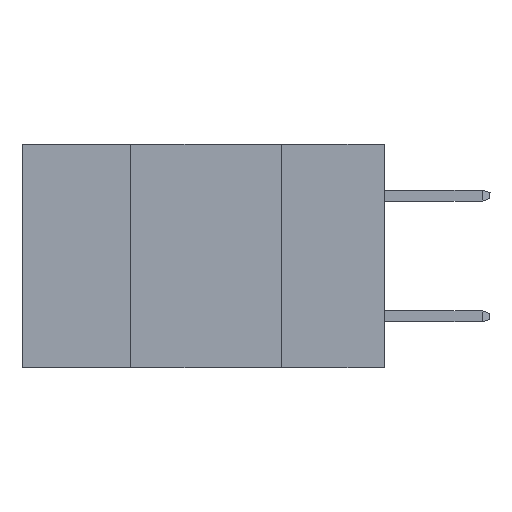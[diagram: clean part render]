
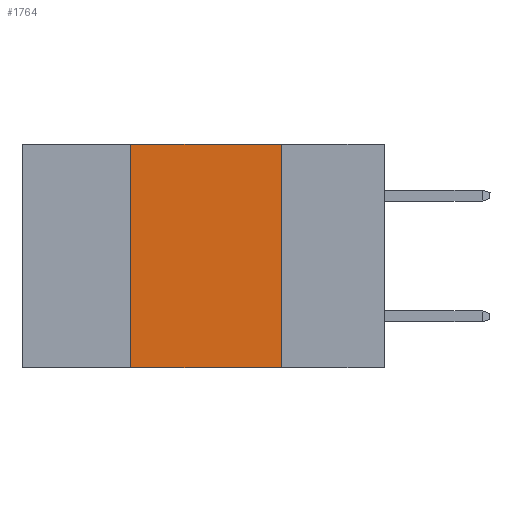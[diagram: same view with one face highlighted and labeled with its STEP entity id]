
A CAD part, left-side view. The second image highlights one B-rep face of the part: STEP entity #1764.
In plain terms, the highlighted planar face has unit normal (-1, 0, 0).
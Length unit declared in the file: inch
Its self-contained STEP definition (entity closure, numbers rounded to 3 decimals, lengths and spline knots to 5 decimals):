
#1295 = VERTEX_POINT ( 'NONE', #20306 ) ;
#1764 = ADVANCED_FACE ( 'NONE', ( #6609 ), #15879, .F. ) ;
#3028 = CARTESIAN_POINT ( 'NONE',  ( 0., 0.17, -0.37 ) ) ;
#3430 = ORIENTED_EDGE ( 'NONE', *, *, #4189, .F. ) ;
#3441 = CARTESIAN_POINT ( 'NONE',  ( 0., 0.42, -0.37 ) ) ;
#4189 = EDGE_CURVE ( 'NONE', #1295, #16465, #11173, .T. ) ;
#4490 = DIRECTION ( 'NONE',  ( 0., 0., -1. ) ) ;
#4942 = DIRECTION ( 'NONE',  ( 0., 0., 1. ) ) ;
#6105 = CARTESIAN_POINT ( 'NONE',  ( 0., 0.6, 0. ) ) ;
#6609 = FACE_OUTER_BOUND ( 'NONE', #9655, .T. ) ;
#7388 = VERTEX_POINT ( 'NONE', #3441 ) ;
#8263 = EDGE_CURVE ( 'NONE', #16465, #20107, #13062, .T. ) ;
#9372 = DIRECTION ( 'NONE',  ( 0., -1., 0. ) ) ;
#9398 = DIRECTION ( 'NONE',  ( 1., 0., 0. ) ) ;
#9655 = EDGE_LOOP ( 'NONE', ( #11807, #3430, #15293, #12681 ) ) ;
#11173 = LINE ( 'NONE', #16276, #14971 ) ;
#11354 = EDGE_CURVE ( 'NONE', #7388, #20107, #13996, .T. ) ;
#11807 = ORIENTED_EDGE ( 'NONE', *, *, #8263, .F. ) ;
#12681 = ORIENTED_EDGE ( 'NONE', *, *, #11354, .T. ) ;
#13062 = LINE ( 'NONE', #14237, #15875 ) ;
#13179 = VECTOR ( 'NONE', #4942, 39.37008 ) ;
#13996 = LINE ( 'NONE', #20866, #19859 ) ;
#14074 = CARTESIAN_POINT ( 'NONE',  ( 0., 0.17, 0. ) ) ;
#14237 = CARTESIAN_POINT ( 'NONE',  ( 0., 0.17, 0. ) ) ;
#14971 = VECTOR ( 'NONE', #20879, 39.37008 ) ;
#15293 = ORIENTED_EDGE ( 'NONE', *, *, #18294, .F. ) ;
#15875 = VECTOR ( 'NONE', #4490, 39.37008 ) ;
#15879 = PLANE ( 'NONE',  #19174 ) ;
#16276 = CARTESIAN_POINT ( 'NONE',  ( 0., 0.6, 0. ) ) ;
#16465 = VERTEX_POINT ( 'NONE', #14074 ) ;
#17513 = DIRECTION ( 'NONE',  ( 0., 0., -1. ) ) ;
#18294 = EDGE_CURVE ( 'NONE', #7388, #1295, #20793, .T. ) ;
#19153 = CARTESIAN_POINT ( 'NONE',  ( 0., 0.42, 0. ) ) ;
#19174 = AXIS2_PLACEMENT_3D ( 'NONE', #6105, #9398, #17513 ) ;
#19859 = VECTOR ( 'NONE', #9372, 39.37008 ) ;
#20107 = VERTEX_POINT ( 'NONE', #3028 ) ;
#20306 = CARTESIAN_POINT ( 'NONE',  ( 0., 0.42, 0. ) ) ;
#20793 = LINE ( 'NONE', #19153, #13179 ) ;
#20866 = CARTESIAN_POINT ( 'NONE',  ( 0., 0.6, -0.37 ) ) ;
#20879 = DIRECTION ( 'NONE',  ( 0., -1., 0. ) ) ;
